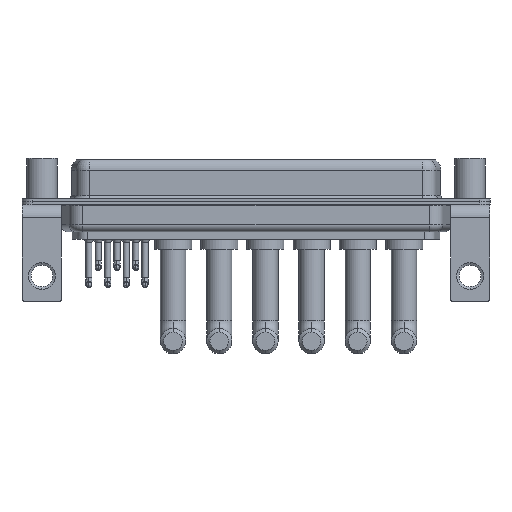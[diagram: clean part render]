
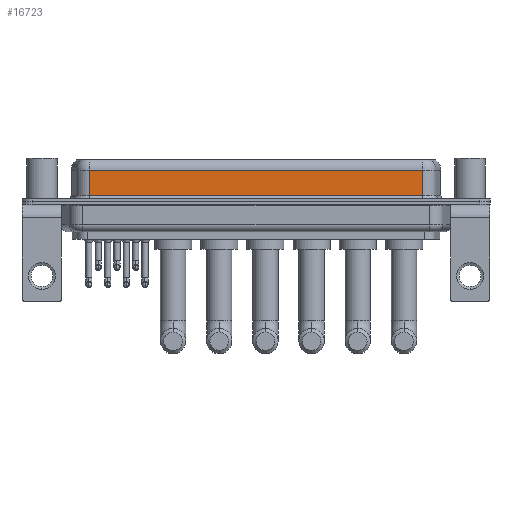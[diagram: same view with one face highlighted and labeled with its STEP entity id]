
A CAD part, front view. The second image highlights one B-rep face of the part: STEP entity #16723.
In plain terms, the highlighted planar face has unit normal (0, -1, 0).
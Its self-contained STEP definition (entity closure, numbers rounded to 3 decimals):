
#515 = DIRECTION ( 'NONE',  ( 0., 1., 0. ) ) ;
#1457 = DIRECTION ( 'NONE',  ( 1., 0., 0. ) ) ;
#1468 = CARTESIAN_POINT ( 'NONE',  ( 7.038, -3.95, 6.4 ) ) ;
#2434 = PLANE ( 'NONE',  #5073 ) ;
#3725 = VECTOR ( 'NONE', #1457, 1000. ) ;
#5073 = AXIS2_PLACEMENT_3D ( 'NONE', #16732, #515, #20114 ) ;
#5932 = CARTESIAN_POINT ( 'NONE',  ( 7.038, -3.95, 0.9 ) ) ;
#5954 = EDGE_LOOP ( 'NONE', ( #8354, #16114, #10308, #16600 ) ) ;
#6252 = LINE ( 'NONE', #1468, #8565 ) ;
#7376 = VECTOR ( 'NONE', #19522, 1000. ) ;
#7605 = CARTESIAN_POINT ( 'NONE',  ( 7.038, -3.95, 4.65 ) ) ;
#8354 = ORIENTED_EDGE ( 'NONE', *, *, #19150, .F. ) ;
#8565 = VECTOR ( 'NONE', #13050, 1000. ) ;
#8860 = EDGE_CURVE ( 'NONE', #11296, #14927, #6252, .T. ) ;
#8873 = EDGE_CURVE ( 'NONE', #19684, #11296, #12733, .T. ) ;
#9608 = CARTESIAN_POINT ( 'NONE',  ( 56.462, -3.95, 6.4 ) ) ;
#10308 = ORIENTED_EDGE ( 'NONE', *, *, #8860, .T. ) ;
#11296 = VERTEX_POINT ( 'NONE', #7605 ) ;
#11441 = CARTESIAN_POINT ( 'NONE',  ( 56.462, -3.95, 0.9 ) ) ;
#12099 = FACE_OUTER_BOUND ( 'NONE', #5954, .T. ) ;
#12733 = LINE ( 'NONE', #14524, #12966 ) ;
#12966 = VECTOR ( 'NONE', #14417, 1000. ) ;
#13050 = DIRECTION ( 'NONE',  ( 0., 0., -1. ) ) ;
#13078 = CARTESIAN_POINT ( 'NONE',  ( 56.462, -3.95, 4.65 ) ) ;
#13134 = LINE ( 'NONE', #11441, #3725 ) ;
#13700 = EDGE_CURVE ( 'NONE', #14927, #14422, #13134, .T. ) ;
#14417 = DIRECTION ( 'NONE',  ( -1., 0., 0. ) ) ;
#14422 = VERTEX_POINT ( 'NONE', #17297 ) ;
#14524 = CARTESIAN_POINT ( 'NONE',  ( 56.462, -3.95, 4.65 ) ) ;
#14927 = VERTEX_POINT ( 'NONE', #5932 ) ;
#15831 = LINE ( 'NONE', #9608, #7376 ) ;
#16114 = ORIENTED_EDGE ( 'NONE', *, *, #8873, .T. ) ;
#16600 = ORIENTED_EDGE ( 'NONE', *, *, #13700, .T. ) ;
#16723 = ADVANCED_FACE ( 'NONE', ( #12099 ), #2434, .F. ) ;
#16732 = CARTESIAN_POINT ( 'NONE',  ( 56.462, -3.95, 6.4 ) ) ;
#17297 = CARTESIAN_POINT ( 'NONE',  ( 56.462, -3.95, 0.9 ) ) ;
#19150 = EDGE_CURVE ( 'NONE', #19684, #14422, #15831, .T. ) ;
#19522 = DIRECTION ( 'NONE',  ( 0., 0., -1. ) ) ;
#19684 = VERTEX_POINT ( 'NONE', #13078 ) ;
#20114 = DIRECTION ( 'NONE',  ( 0., 0., 1. ) ) ;
